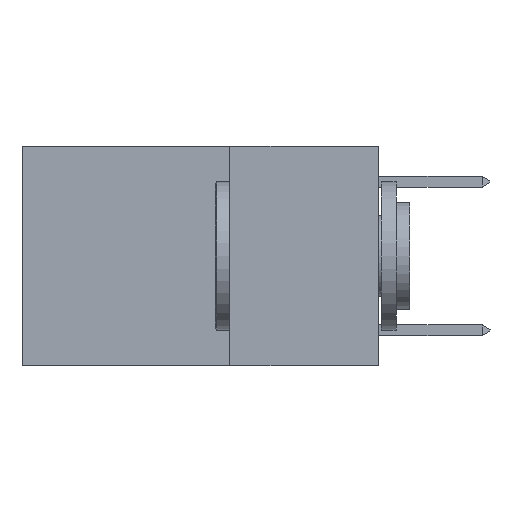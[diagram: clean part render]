
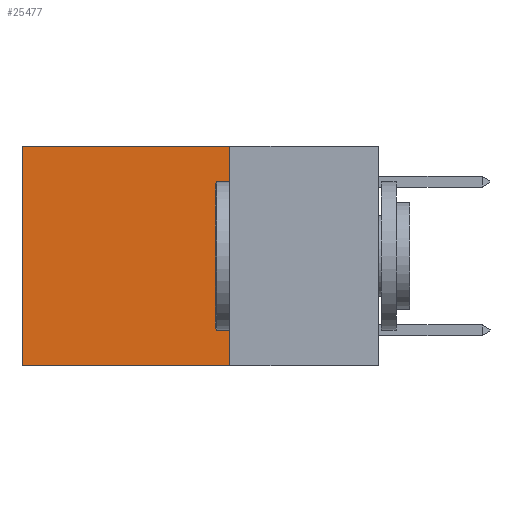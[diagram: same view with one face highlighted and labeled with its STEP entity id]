
A CAD part, left-side view. The second image highlights one B-rep face of the part: STEP entity #25477.
In plain terms, the highlighted planar face has unit normal (-1, 0, 0).
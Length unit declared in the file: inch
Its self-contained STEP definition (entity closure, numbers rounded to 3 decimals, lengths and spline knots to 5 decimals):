
#1226 = DIRECTION ( 'NONE',  ( 0., 0., -1. ) ) ;
#2027 = ORIENTED_EDGE ( 'NONE', *, *, #9567, .T. ) ;
#3284 = ORIENTED_EDGE ( 'NONE', *, *, #24593, .F. ) ;
#3360 = EDGE_CURVE ( 'NONE', #19285, #17526, #26461, .T. ) ;
#4759 = CARTESIAN_POINT ( 'NONE',  ( 0.2625, 0.6, 0. ) ) ;
#5078 = VECTOR ( 'NONE', #18323, 39.37008 ) ;
#5595 = ORIENTED_EDGE ( 'NONE', *, *, #3360, .F. ) ;
#6500 = VECTOR ( 'NONE', #24166, 39.37008 ) ;
#6904 = DIRECTION ( 'NONE',  ( 0., 1., 0. ) ) ;
#8193 = FACE_OUTER_BOUND ( 'NONE', #15143, .T. ) ;
#8847 = DIRECTION ( 'NONE',  ( 0., 0., -1. ) ) ;
#8857 = CARTESIAN_POINT ( 'NONE',  ( 0.2625, 0.25, -0.37 ) ) ;
#9486 = LINE ( 'NONE', #13703, #5078 ) ;
#9567 = EDGE_CURVE ( 'NONE', #22250, #28384, #15497, .T. ) ;
#10575 = CARTESIAN_POINT ( 'NONE',  ( 0.2625, 0.6, 0. ) ) ;
#10638 = VECTOR ( 'NONE', #6904, 39.37008 ) ;
#11016 = EDGE_CURVE ( 'NONE', #28384, #17526, #26216, .T. ) ;
#12752 = CARTESIAN_POINT ( 'NONE',  ( 0.2625, 0.25, 0. ) ) ;
#13703 = CARTESIAN_POINT ( 'NONE',  ( 0.2625, 0.25, 0. ) ) ;
#14394 = VECTOR ( 'NONE', #8847, 39.37008 ) ;
#14735 = CARTESIAN_POINT ( 'NONE',  ( 0.2625, 0.25, 0. ) ) ;
#15143 = EDGE_LOOP ( 'NONE', ( #22423, #5595, #3284, #2027 ) ) ;
#15497 = LINE ( 'NONE', #12752, #6500 ) ;
#17031 = PLANE ( 'NONE',  #17600 ) ;
#17526 = VERTEX_POINT ( 'NONE', #22874 ) ;
#17600 = AXIS2_PLACEMENT_3D ( 'NONE', #14735, #27743, #1226 ) ;
#18323 = DIRECTION ( 'NONE',  ( 0., 0., -1. ) ) ;
#19285 = VERTEX_POINT ( 'NONE', #8857 ) ;
#22250 = VERTEX_POINT ( 'NONE', #24187 ) ;
#22423 = ORIENTED_EDGE ( 'NONE', *, *, #11016, .T. ) ;
#22874 = CARTESIAN_POINT ( 'NONE',  ( 0.2625, 0.6, -0.37 ) ) ;
#24166 = DIRECTION ( 'NONE',  ( 0., 1., 0. ) ) ;
#24187 = CARTESIAN_POINT ( 'NONE',  ( 0.2625, 0.25, 0. ) ) ;
#24593 = EDGE_CURVE ( 'NONE', #22250, #19285, #9486, .T. ) ;
#25477 = ADVANCED_FACE ( 'NONE', ( #8193 ), #17031, .F. ) ;
#26216 = LINE ( 'NONE', #10575, #14394 ) ;
#26461 = LINE ( 'NONE', #26716, #10638 ) ;
#26716 = CARTESIAN_POINT ( 'NONE',  ( 0.2625, 0.25, -0.37 ) ) ;
#27743 = DIRECTION ( 'NONE',  ( 1., 0., 0. ) ) ;
#28384 = VERTEX_POINT ( 'NONE', #4759 ) ;
